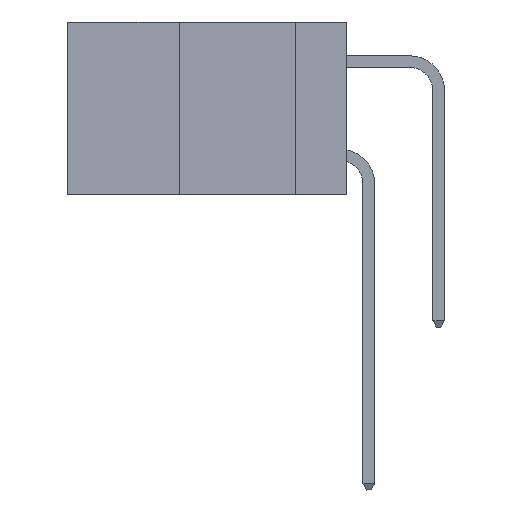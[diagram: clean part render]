
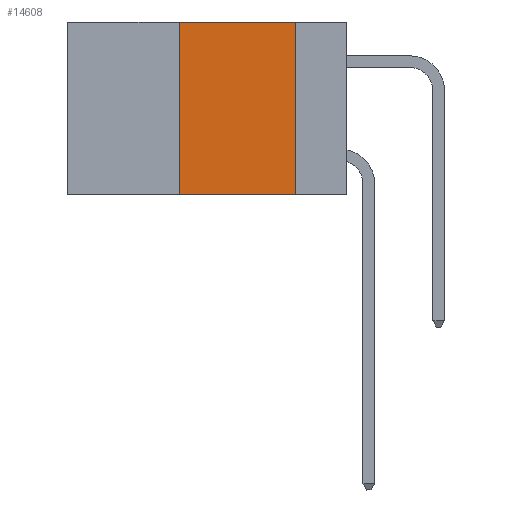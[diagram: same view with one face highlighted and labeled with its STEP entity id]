
A CAD part, left-side view. The second image highlights one B-rep face of the part: STEP entity #14608.
In plain terms, the highlighted planar face has unit normal (-1, 0, 0).
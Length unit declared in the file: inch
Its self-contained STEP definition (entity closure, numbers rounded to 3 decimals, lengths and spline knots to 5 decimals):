
#1118 = VECTOR ( 'NONE', #17739, 39.37008 ) ;
#1694 = VERTEX_POINT ( 'NONE', #6555 ) ;
#1788 = DIRECTION ( 'NONE',  ( 0., -1., 0. ) ) ;
#2235 = VERTEX_POINT ( 'NONE', #11173 ) ;
#2323 = DIRECTION ( 'NONE',  ( 1., 0., 0. ) ) ;
#2546 = LINE ( 'NONE', #12577, #17562 ) ;
#2702 = CARTESIAN_POINT ( 'NONE',  ( 0., 0.6, -0.37 ) ) ;
#3400 = CARTESIAN_POINT ( 'NONE',  ( 0., 0.11, 0. ) ) ;
#3449 = DIRECTION ( 'NONE',  ( 0., 0., 1. ) ) ;
#5209 = LINE ( 'NONE', #2702, #1118 ) ;
#5615 = LINE ( 'NONE', #13601, #15373 ) ;
#6091 = ORIENTED_EDGE ( 'NONE', *, *, #9011, .F. ) ;
#6555 = CARTESIAN_POINT ( 'NONE',  ( 0., 0.36, -0.37 ) ) ;
#7134 = LINE ( 'NONE', #12456, #10742 ) ;
#7955 = EDGE_CURVE ( 'NONE', #8010, #2235, #7134, .T. ) ;
#7970 = EDGE_LOOP ( 'NONE', ( #9142, #19365, #6091, #14382 ) ) ;
#8010 = VERTEX_POINT ( 'NONE', #3400 ) ;
#8478 = EDGE_CURVE ( 'NONE', #1694, #2235, #5209, .T. ) ;
#8663 = PLANE ( 'NONE',  #12415 ) ;
#9011 = EDGE_CURVE ( 'NONE', #1694, #14542, #2546, .T. ) ;
#9142 = ORIENTED_EDGE ( 'NONE', *, *, #7955, .F. ) ;
#9925 = EDGE_CURVE ( 'NONE', #14542, #8010, #5615, .T. ) ;
#10103 = CARTESIAN_POINT ( 'NONE',  ( 0., 0.36, 0. ) ) ;
#10711 = DIRECTION ( 'NONE',  ( 0., 0., -1. ) ) ;
#10742 = VECTOR ( 'NONE', #10711, 39.37008 ) ;
#11173 = CARTESIAN_POINT ( 'NONE',  ( 0., 0.11, -0.37 ) ) ;
#11295 = FACE_OUTER_BOUND ( 'NONE', #7970, .T. ) ;
#12415 = AXIS2_PLACEMENT_3D ( 'NONE', #17821, #2323, #13120 ) ;
#12456 = CARTESIAN_POINT ( 'NONE',  ( 0., 0.11, 0. ) ) ;
#12577 = CARTESIAN_POINT ( 'NONE',  ( 0., 0.36, 0. ) ) ;
#13120 = DIRECTION ( 'NONE',  ( 0., 0., -1. ) ) ;
#13601 = CARTESIAN_POINT ( 'NONE',  ( 0., 0.6, 0. ) ) ;
#14382 = ORIENTED_EDGE ( 'NONE', *, *, #8478, .T. ) ;
#14542 = VERTEX_POINT ( 'NONE', #10103 ) ;
#14608 = ADVANCED_FACE ( 'NONE', ( #11295 ), #8663, .F. ) ;
#15373 = VECTOR ( 'NONE', #1788, 39.37008 ) ;
#17562 = VECTOR ( 'NONE', #3449, 39.37008 ) ;
#17739 = DIRECTION ( 'NONE',  ( 0., -1., 0. ) ) ;
#17821 = CARTESIAN_POINT ( 'NONE',  ( 0., 0.6, 0. ) ) ;
#19365 = ORIENTED_EDGE ( 'NONE', *, *, #9925, .F. ) ;
